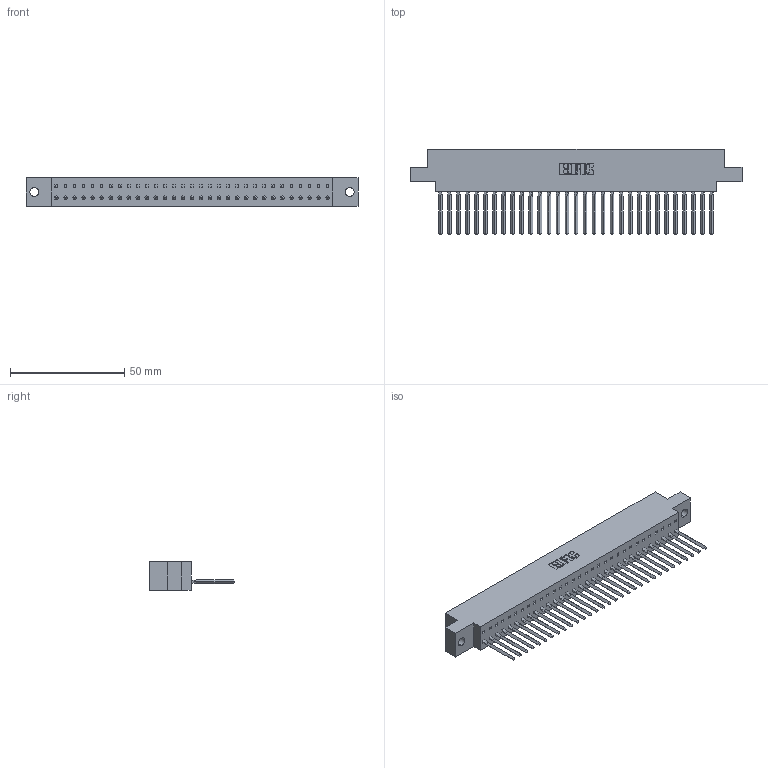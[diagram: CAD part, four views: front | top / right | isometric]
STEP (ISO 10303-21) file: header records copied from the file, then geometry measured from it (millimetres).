
FILE_DESCRIPTION (( 'STEP AP203' ), '1' );
FILE_NAME ('317-031-541-604.STEP', '2020-02-27T20:47:08', ( '' ), ( '' ), 'SwSTEP 2.0', 'SolidWorks 2016', '' );
FILE_SCHEMA (( 'CONFIG_CONTROL_DESIGN' ));
Length unit declared in the file: inch
Products named in the file (3): 317-290-002_541; 317-031-541-604; 317 Part_.156 Dia - TH
Assembly tree (32 placements, depth 2):
  317-031-541-604
    317 Part_.156 Dia - TH
    317-290-002_541  x31
Bounding box: 145.54 x 37.34 x 12.7 mm (x, y, z)
Volume: 23175.9 mm3; surface area: 32200.4 mm2
Topology: 32 solids, 32 shells, 4814 faces, 13729 edges, 8924 vertices
Faces by surface type: plane 3902, cylinder 788, bspline 124
Entity records: 46904 total; most frequent: CARTESIAN_POINT 8974, ORIENTED_EDGE 8258, DIRECTION 6775, EDGE_CURVE 4129, LINE 3765, VECTOR 3765, VERTEX_POINT 2744, AXIS2_PLACEMENT_3D 1505
